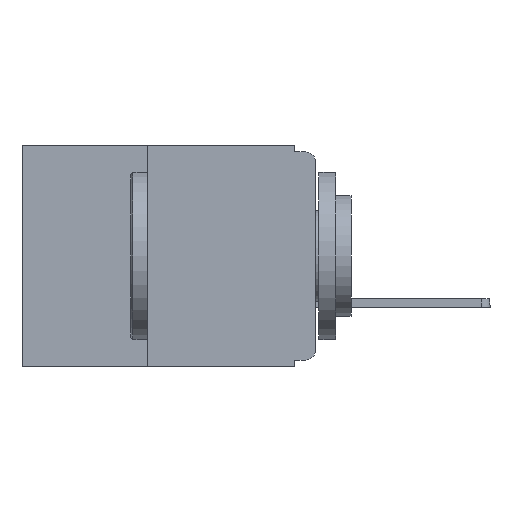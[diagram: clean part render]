
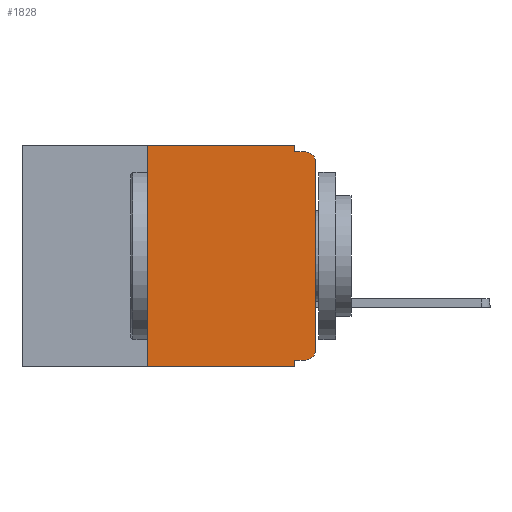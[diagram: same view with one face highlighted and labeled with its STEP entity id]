
A CAD part, left-side view. The second image highlights one B-rep face of the part: STEP entity #1828.
In plain terms, the highlighted planar face has unit normal (-1, 0, 0).
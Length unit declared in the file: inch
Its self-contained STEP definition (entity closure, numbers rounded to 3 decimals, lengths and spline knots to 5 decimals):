
#423 = VERTEX_POINT ( 'NONE', #4924 ) ;
#1238 = PLANE ( 'NONE',  #14824 ) ;
#1761 = ORIENTED_EDGE ( 'NONE', *, *, #4729, .T. ) ;
#1828 = ADVANCED_FACE ( 'NONE', ( #3104 ), #1238, .F. ) ;
#2001 = VERTEX_POINT ( 'NONE', #8295 ) ;
#2444 = CARTESIAN_POINT ( 'NONE',  ( 0., 0., -0.32 ) ) ;
#2737 = ORIENTED_EDGE ( 'NONE', *, *, #18913, .T. ) ;
#2919 = ORIENTED_EDGE ( 'NONE', *, *, #4035, .F. ) ;
#3104 = FACE_OUTER_BOUND ( 'NONE', #17237, .T. ) ;
#3176 = CIRCLE ( 'NONE', #14297, 0.015 ) ;
#3228 = ORIENTED_EDGE ( 'NONE', *, *, #8127, .F. ) ;
#3251 = ORIENTED_EDGE ( 'NONE', *, *, #16351, .F. ) ;
#3295 = ORIENTED_EDGE ( 'NONE', *, *, #14863, .F. ) ;
#3657 = ORIENTED_EDGE ( 'NONE', *, *, #15197, .T. ) ;
#3702 = ORIENTED_EDGE ( 'NONE', *, *, #16855, .F. ) ;
#3765 = ORIENTED_EDGE ( 'NONE', *, *, #9281, .F. ) ;
#4035 = EDGE_CURVE ( 'NONE', #10932, #16000, #15342, .T. ) ;
#4054 = VERTEX_POINT ( 'NONE', #16505 ) ;
#4167 = ORIENTED_EDGE ( 'NONE', *, *, #8925, .T. ) ;
#4371 = VECTOR ( 'NONE', #6160, 39.37008 ) ;
#4622 = LINE ( 'NONE', #6977, #4371 ) ;
#4729 = EDGE_CURVE ( 'NONE', #18532, #9206, #13170, .T. ) ;
#4872 = CARTESIAN_POINT ( 'NONE',  ( 0., 0.015, -0.025 ) ) ;
#4924 = CARTESIAN_POINT ( 'NONE',  ( 0., 0.015, -0.32 ) ) ;
#5135 = VECTOR ( 'NONE', #17209, 39.37008 ) ;
#5343 = DIRECTION ( 'NONE',  ( 0., 0., -1. ) ) ;
#5372 = DIRECTION ( 'NONE',  ( -1., 0., 0. ) ) ;
#5423 = CARTESIAN_POINT ( 'NONE',  ( 0., 0.015, -0.305 ) ) ;
#5531 = VERTEX_POINT ( 'NONE', #18371 ) ;
#5609 = VERTEX_POINT ( 'NONE', #11201 ) ;
#6160 = DIRECTION ( 'NONE',  ( 0., 0., -1. ) ) ;
#6921 = VECTOR ( 'NONE', #14905, 39.37008 ) ;
#6977 = CARTESIAN_POINT ( 'NONE',  ( 0., 0.031, -0.33 ) ) ;
#6979 = VECTOR ( 'NONE', #18878, 39.37008 ) ;
#7034 = CARTESIAN_POINT ( 'NONE',  ( 0., 0., -0.025 ) ) ;
#7090 = LINE ( 'NONE', #2444, #6979 ) ;
#7301 = LINE ( 'NONE', #14961, #6921 ) ;
#8127 = EDGE_CURVE ( 'NONE', #5609, #10932, #13549, .T. ) ;
#8295 = CARTESIAN_POINT ( 'NONE',  ( 0., 0.25, 0. ) ) ;
#8475 = CIRCLE ( 'NONE', #18230, 0.015 ) ;
#8767 = CARTESIAN_POINT ( 'NONE',  ( 0., 0.031, 0. ) ) ;
#8836 = DIRECTION ( 'NONE',  ( 0., 0., -1. ) ) ;
#8925 = EDGE_CURVE ( 'NONE', #423, #18532, #8475, .T. ) ;
#8949 = CARTESIAN_POINT ( 'NONE',  ( 0., 0.031, -0.01 ) ) ;
#8952 = CARTESIAN_POINT ( 'NONE',  ( 0., 0.25, -0.33 ) ) ;
#9033 = CARTESIAN_POINT ( 'NONE',  ( 0., 0.437, 0. ) ) ;
#9076 = DIRECTION ( 'NONE',  ( 0., 0., 1. ) ) ;
#9206 = VERTEX_POINT ( 'NONE', #7034 ) ;
#9281 = EDGE_CURVE ( 'NONE', #423, #4054, #7090, .T. ) ;
#9526 = VERTEX_POINT ( 'NONE', #13674 ) ;
#10932 = VERTEX_POINT ( 'NONE', #8949 ) ;
#11201 = CARTESIAN_POINT ( 'NONE',  ( 0., 0.031, 0. ) ) ;
#12470 = DIRECTION ( 'NONE',  ( 0., -1., 0. ) ) ;
#12652 = CARTESIAN_POINT ( 'NONE',  ( 0., 0.437, -0.33 ) ) ;
#13170 = LINE ( 'NONE', #14787, #13171 ) ;
#13171 = VECTOR ( 'NONE', #14514, 39.37008 ) ;
#13261 = DIRECTION ( 'NONE',  ( 0., 0., -1. ) ) ;
#13549 = LINE ( 'NONE', #8767, #13766 ) ;
#13674 = CARTESIAN_POINT ( 'NONE',  ( 0., 0.031, -0.33 ) ) ;
#13766 = VECTOR ( 'NONE', #8836, 39.37008 ) ;
#14297 = AXIS2_PLACEMENT_3D ( 'NONE', #4872, #18455, #14394 ) ;
#14323 = VECTOR ( 'NONE', #12470, 39.37008 ) ;
#14343 = LINE ( 'NONE', #12652, #14323 ) ;
#14394 = DIRECTION ( 'NONE',  ( 0., 0., -1. ) ) ;
#14514 = DIRECTION ( 'NONE',  ( 0., 0., 1. ) ) ;
#14787 = CARTESIAN_POINT ( 'NONE',  ( 0., 0., 0. ) ) ;
#14824 = AXIS2_PLACEMENT_3D ( 'NONE', #9033, #17765, #13261 ) ;
#14863 = EDGE_CURVE ( 'NONE', #5531, #2001, #16747, .T. ) ;
#14905 = DIRECTION ( 'NONE',  ( 0., -1., 0. ) ) ;
#14961 = CARTESIAN_POINT ( 'NONE',  ( 0., 0.437, 0. ) ) ;
#15197 = EDGE_CURVE ( 'NONE', #5531, #9526, #14343, .T. ) ;
#15342 = LINE ( 'NONE', #17767, #5135 ) ;
#16000 = VERTEX_POINT ( 'NONE', #19021 ) ;
#16351 = EDGE_CURVE ( 'NONE', #2001, #5609, #7301, .T. ) ;
#16505 = CARTESIAN_POINT ( 'NONE',  ( 0., 0.031, -0.32 ) ) ;
#16666 = VECTOR ( 'NONE', #9076, 39.37008 ) ;
#16747 = LINE ( 'NONE', #8952, #16666 ) ;
#16855 = EDGE_CURVE ( 'NONE', #4054, #9526, #4622, .T. ) ;
#17209 = DIRECTION ( 'NONE',  ( 0., -1., 0. ) ) ;
#17237 = EDGE_LOOP ( 'NONE', ( #1761, #2737, #2919, #3228, #3251, #3295, #3657, #3702, #3765, #4167 ) ) ;
#17765 = DIRECTION ( 'NONE',  ( 1., 0., 0. ) ) ;
#17767 = CARTESIAN_POINT ( 'NONE',  ( 0., 0., -0.01 ) ) ;
#17803 = CARTESIAN_POINT ( 'NONE',  ( 0., 0., -0.305 ) ) ;
#18230 = AXIS2_PLACEMENT_3D ( 'NONE', #5423, #5372, #5343 ) ;
#18371 = CARTESIAN_POINT ( 'NONE',  ( 0., 0.25, -0.33 ) ) ;
#18455 = DIRECTION ( 'NONE',  ( -1., 0., 0. ) ) ;
#18532 = VERTEX_POINT ( 'NONE', #17803 ) ;
#18878 = DIRECTION ( 'NONE',  ( 0., 1., 0. ) ) ;
#18913 = EDGE_CURVE ( 'NONE', #9206, #16000, #3176, .T. ) ;
#19021 = CARTESIAN_POINT ( 'NONE',  ( 0., 0.015, -0.01 ) ) ;
